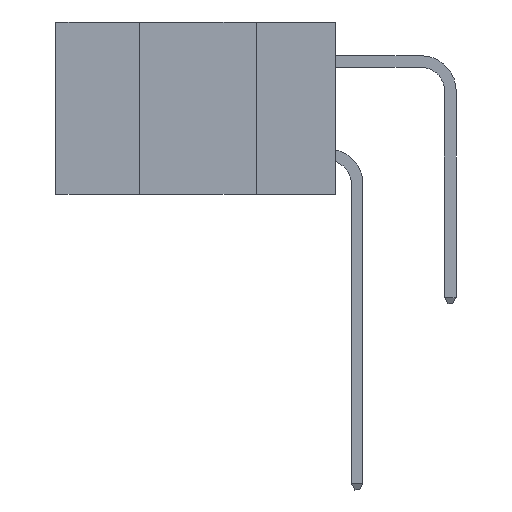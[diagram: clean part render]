
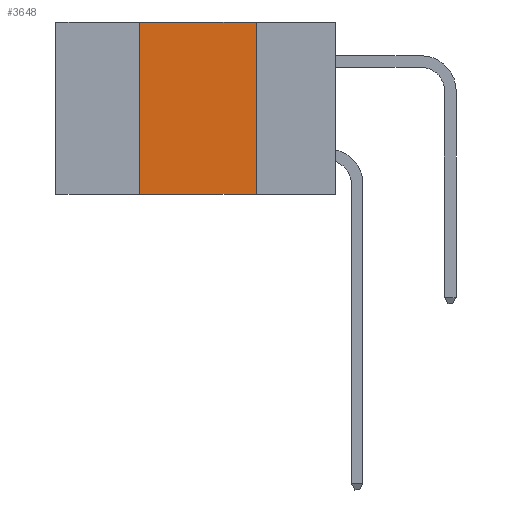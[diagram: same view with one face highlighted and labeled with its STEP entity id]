
A CAD part, left-side view. The second image highlights one B-rep face of the part: STEP entity #3648.
In plain terms, the highlighted planar face has unit normal (-1, 0, 0).
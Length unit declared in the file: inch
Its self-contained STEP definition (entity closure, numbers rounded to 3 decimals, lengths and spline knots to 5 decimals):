
#482 = DIRECTION ( 'NONE',  ( 0., 0., -1. ) ) ;
#493 = ORIENTED_EDGE ( 'NONE', *, *, #9587, .F. ) ;
#848 = CARTESIAN_POINT ( 'NONE',  ( 0., 0.17, 0. ) ) ;
#863 = CARTESIAN_POINT ( 'NONE',  ( 0., 0.17, -0.37 ) ) ;
#1281 = VECTOR ( 'NONE', #3784, 39.37008 ) ;
#1319 = CARTESIAN_POINT ( 'NONE',  ( 0., 0.6, 0. ) ) ;
#1368 = VECTOR ( 'NONE', #2273, 39.37008 ) ;
#1470 = FACE_OUTER_BOUND ( 'NONE', #11193, .T. ) ;
#1622 = VECTOR ( 'NONE', #9951, 39.37008 ) ;
#2172 = LINE ( 'NONE', #4928, #10791 ) ;
#2272 = ORIENTED_EDGE ( 'NONE', *, *, #6344, .T. ) ;
#2273 = DIRECTION ( 'NONE',  ( 0., -1., 0. ) ) ;
#2848 = CARTESIAN_POINT ( 'NONE',  ( 0., 0.42, -0.37 ) ) ;
#2955 = CARTESIAN_POINT ( 'NONE',  ( 0., 0.6, 0. ) ) ;
#3010 = AXIS2_PLACEMENT_3D ( 'NONE', #2955, #6306, #482 ) ;
#3405 = EDGE_CURVE ( 'NONE', #8235, #3989, #4012, .T. ) ;
#3527 = CARTESIAN_POINT ( 'NONE',  ( 0., 0.17, 0. ) ) ;
#3648 = ADVANCED_FACE ( 'NONE', ( #1470 ), #10073, .F. ) ;
#3784 = DIRECTION ( 'NONE',  ( 0., 0., 1. ) ) ;
#3863 = CARTESIAN_POINT ( 'NONE',  ( 0., 0.42, 0. ) ) ;
#3989 = VERTEX_POINT ( 'NONE', #863 ) ;
#4012 = LINE ( 'NONE', #3527, #1622 ) ;
#4042 = LINE ( 'NONE', #1319, #1368 ) ;
#4928 = CARTESIAN_POINT ( 'NONE',  ( 0., 0.6, -0.37 ) ) ;
#5079 = DIRECTION ( 'NONE',  ( 0., -1., 0. ) ) ;
#6051 = ORIENTED_EDGE ( 'NONE', *, *, #6396, .F. ) ;
#6306 = DIRECTION ( 'NONE',  ( 1., 0., 0. ) ) ;
#6344 = EDGE_CURVE ( 'NONE', #9235, #3989, #2172, .T. ) ;
#6396 = EDGE_CURVE ( 'NONE', #9235, #8116, #8670, .T. ) ;
#8116 = VERTEX_POINT ( 'NONE', #11034 ) ;
#8235 = VERTEX_POINT ( 'NONE', #848 ) ;
#8670 = LINE ( 'NONE', #3863, #1281 ) ;
#9235 = VERTEX_POINT ( 'NONE', #2848 ) ;
#9587 = EDGE_CURVE ( 'NONE', #8116, #8235, #4042, .T. ) ;
#9951 = DIRECTION ( 'NONE',  ( 0., 0., -1. ) ) ;
#10073 = PLANE ( 'NONE',  #3010 ) ;
#10791 = VECTOR ( 'NONE', #5079, 39.37008 ) ;
#10881 = ORIENTED_EDGE ( 'NONE', *, *, #3405, .F. ) ;
#11034 = CARTESIAN_POINT ( 'NONE',  ( 0., 0.42, 0. ) ) ;
#11193 = EDGE_LOOP ( 'NONE', ( #10881, #493, #6051, #2272 ) ) ;
